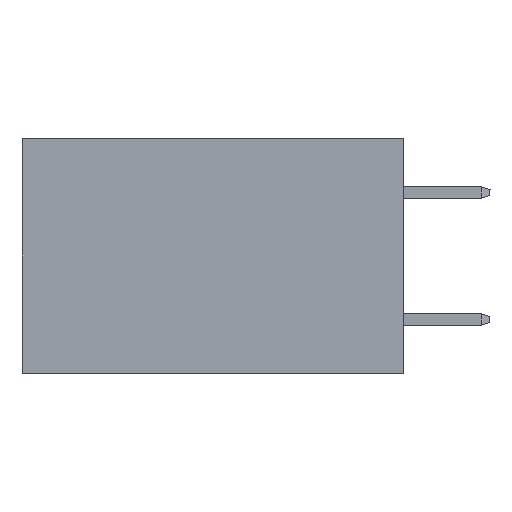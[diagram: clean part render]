
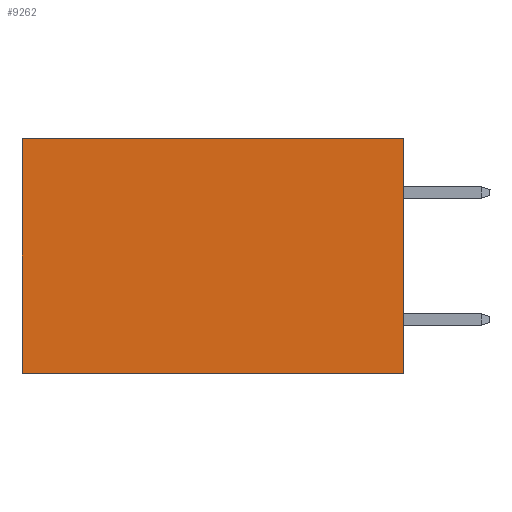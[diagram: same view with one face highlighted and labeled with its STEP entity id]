
A CAD part, left-side view. The second image highlights one B-rep face of the part: STEP entity #9262.
In plain terms, the highlighted planar face has unit normal (-1, 0, 0).
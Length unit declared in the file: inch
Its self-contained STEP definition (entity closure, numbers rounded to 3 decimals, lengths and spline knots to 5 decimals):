
#85 = DIRECTION ( 'NONE',  ( 1., 0., 0. ) ) ;
#371 = EDGE_LOOP ( 'NONE', ( #20376, #1358, #15682, #3728 ) ) ;
#545 = FACE_OUTER_BOUND ( 'NONE', #371, .T. ) ;
#1358 = ORIENTED_EDGE ( 'NONE', *, *, #13893, .F. ) ;
#1444 = VERTEX_POINT ( 'NONE', #14224 ) ;
#3027 = CARTESIAN_POINT ( 'NONE',  ( 0.2875, 0., 0. ) ) ;
#3108 = CARTESIAN_POINT ( 'NONE',  ( 0.2875, 0., 0. ) ) ;
#3728 = ORIENTED_EDGE ( 'NONE', *, *, #10355, .T. ) ;
#3837 = LINE ( 'NONE', #8133, #8120 ) ;
#4078 = CARTESIAN_POINT ( 'NONE',  ( 0.2875, 0., 0. ) ) ;
#4269 = VECTOR ( 'NONE', #6688, 39.37008 ) ;
#4746 = LINE ( 'NONE', #3027, #4269 ) ;
#5393 = VERTEX_POINT ( 'NONE', #21150 ) ;
#5425 = CARTESIAN_POINT ( 'NONE',  ( 0.2875, 0.6, -0.37 ) ) ;
#6688 = DIRECTION ( 'NONE',  ( 0., 0., -1. ) ) ;
#7065 = DIRECTION ( 'NONE',  ( 0., 0., -1. ) ) ;
#8120 = VECTOR ( 'NONE', #13151, 39.37008 ) ;
#8133 = CARTESIAN_POINT ( 'NONE',  ( 0.2875, 0., -0.37 ) ) ;
#9262 = ADVANCED_FACE ( 'NONE', ( #545 ), #14441, .F. ) ;
#9709 = CARTESIAN_POINT ( 'NONE',  ( 0.2875, 0., 0. ) ) ;
#9911 = VECTOR ( 'NONE', #9976, 39.37008 ) ;
#9961 = AXIS2_PLACEMENT_3D ( 'NONE', #4078, #85, #7065 ) ;
#9976 = DIRECTION ( 'NONE',  ( 0., 1., 0. ) ) ;
#10355 = EDGE_CURVE ( 'NONE', #10625, #5393, #13352, .T. ) ;
#10625 = VERTEX_POINT ( 'NONE', #9709 ) ;
#10661 = VECTOR ( 'NONE', #18602, 39.37008 ) ;
#10765 = EDGE_CURVE ( 'NONE', #5393, #19702, #11803, .T. ) ;
#11803 = LINE ( 'NONE', #22285, #10661 ) ;
#13151 = DIRECTION ( 'NONE',  ( 0., 1., 0. ) ) ;
#13352 = LINE ( 'NONE', #3108, #9911 ) ;
#13893 = EDGE_CURVE ( 'NONE', #1444, #19702, #3837, .T. ) ;
#14224 = CARTESIAN_POINT ( 'NONE',  ( 0.2875, 0., -0.37 ) ) ;
#14441 = PLANE ( 'NONE',  #9961 ) ;
#15682 = ORIENTED_EDGE ( 'NONE', *, *, #16923, .F. ) ;
#16923 = EDGE_CURVE ( 'NONE', #10625, #1444, #4746, .T. ) ;
#18602 = DIRECTION ( 'NONE',  ( 0., 0., -1. ) ) ;
#19702 = VERTEX_POINT ( 'NONE', #5425 ) ;
#20376 = ORIENTED_EDGE ( 'NONE', *, *, #10765, .T. ) ;
#21150 = CARTESIAN_POINT ( 'NONE',  ( 0.2875, 0.6, 0. ) ) ;
#22285 = CARTESIAN_POINT ( 'NONE',  ( 0.2875, 0.6, 0. ) ) ;
